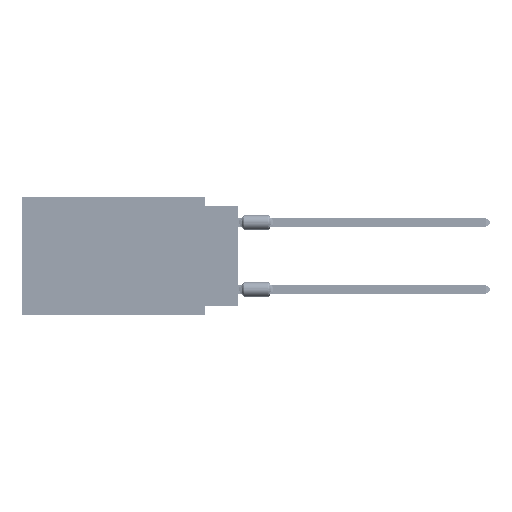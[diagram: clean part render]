
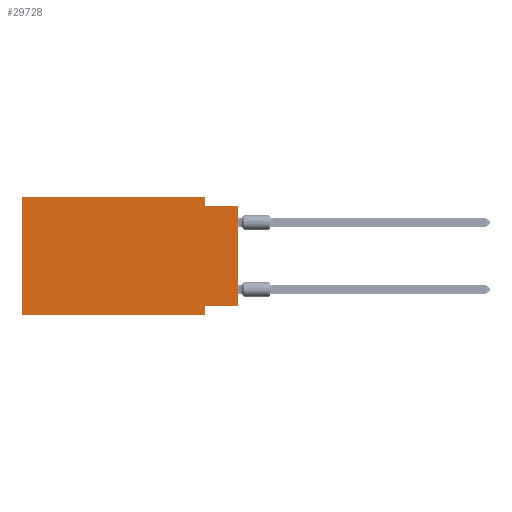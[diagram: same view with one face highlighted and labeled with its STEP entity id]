
A CAD part, left-side view. The second image highlights one B-rep face of the part: STEP entity #29728.
In plain terms, the highlighted planar face has unit normal (-1, 0, 0).
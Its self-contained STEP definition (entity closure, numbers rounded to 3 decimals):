
#1535 = VECTOR ( 'NONE', #17177, 1000. ) ;
#1628 = VECTOR ( 'NONE', #31292, 1000. ) ;
#6155 = DIRECTION ( 'NONE',  ( 0., 1., 0. ) ) ;
#7328 = LINE ( 'NONE', #43851, #18279 ) ;
#7484 = CARTESIAN_POINT ( 'NONE',  ( 0., 0., -0.635 ) ) ;
#7489 = LINE ( 'NONE', #72980, #1628 ) ;
#8551 = LINE ( 'NONE', #26423, #54644 ) ;
#9757 = VERTEX_POINT ( 'NONE', #61402 ) ;
#10589 = CARTESIAN_POINT ( 'NONE',  ( 0., 16.383, -8.89 ) ) ;
#12714 = ORIENTED_EDGE ( 'NONE', *, *, #69511, .F. ) ;
#13499 = VERTEX_POINT ( 'NONE', #23601 ) ;
#14620 = CARTESIAN_POINT ( 'NONE',  ( 0., 2.54, -8.255 ) ) ;
#14882 = PLANE ( 'NONE',  #59758 ) ;
#16758 = VERTEX_POINT ( 'NONE', #65951 ) ;
#16774 = VERTEX_POINT ( 'NONE', #60002 ) ;
#17177 = DIRECTION ( 'NONE',  ( 0., 0., 1. ) ) ;
#18279 = VECTOR ( 'NONE', #6155, 1000. ) ;
#19042 = EDGE_CURVE ( 'NONE', #13499, #16774, #39301, .T. ) ;
#19357 = ORIENTED_EDGE ( 'NONE', *, *, #62565, .F. ) ;
#20249 = DIRECTION ( 'NONE',  ( 0., 0., 1. ) ) ;
#22087 = VERTEX_POINT ( 'NONE', #34062 ) ;
#23601 = CARTESIAN_POINT ( 'NONE',  ( 0., 2.54, 0. ) ) ;
#24843 = EDGE_CURVE ( 'NONE', #33202, #16758, #37282, .T. ) ;
#26423 = CARTESIAN_POINT ( 'NONE',  ( 0., 2.54, -8.89 ) ) ;
#27209 = DIRECTION ( 'NONE',  ( 0., 0., -1. ) ) ;
#29728 = ADVANCED_FACE ( 'NONE', ( #76386 ), #14882, .F. ) ;
#31292 = DIRECTION ( 'NONE',  ( 0., -1., 0. ) ) ;
#33150 = DIRECTION ( 'NONE',  ( 1., 0., 0. ) ) ;
#33202 = VERTEX_POINT ( 'NONE', #10589 ) ;
#34062 = CARTESIAN_POINT ( 'NONE',  ( 0., 16.383, 0. ) ) ;
#34700 = ORIENTED_EDGE ( 'NONE', *, *, #24843, .T. ) ;
#37282 = LINE ( 'NONE', #49174, #55577 ) ;
#38123 = CARTESIAN_POINT ( 'NONE',  ( 0., 16.383, 0. ) ) ;
#38376 = VECTOR ( 'NONE', #38894, 1000. ) ;
#38894 = DIRECTION ( 'NONE',  ( 0., -1., 0. ) ) ;
#39301 = LINE ( 'NONE', #50836, #75336 ) ;
#39895 = CARTESIAN_POINT ( 'NONE',  ( 0., 16.383, 0. ) ) ;
#42739 = ORIENTED_EDGE ( 'NONE', *, *, #52417, .F. ) ;
#43851 = CARTESIAN_POINT ( 'NONE',  ( 0., 0., -8.255 ) ) ;
#43977 = EDGE_CURVE ( 'NONE', #16774, #49335, #7489, .T. ) ;
#46890 = ORIENTED_EDGE ( 'NONE', *, *, #19042, .F. ) ;
#47357 = LINE ( 'NONE', #71553, #1535 ) ;
#49139 = VECTOR ( 'NONE', #20249, 1000. ) ;
#49174 = CARTESIAN_POINT ( 'NONE',  ( 0., 16.383, -8.89 ) ) ;
#49312 = ORIENTED_EDGE ( 'NONE', *, *, #43977, .F. ) ;
#49335 = VERTEX_POINT ( 'NONE', #7484 ) ;
#50636 = DIRECTION ( 'NONE',  ( 0., 0., -1. ) ) ;
#50836 = CARTESIAN_POINT ( 'NONE',  ( 0., 2.54, 0. ) ) ;
#52417 = EDGE_CURVE ( 'NONE', #22087, #13499, #69056, .T. ) ;
#54644 = VECTOR ( 'NONE', #27209, 1000. ) ;
#55577 = VECTOR ( 'NONE', #62272, 1000. ) ;
#58422 = EDGE_CURVE ( 'NONE', #9757, #49335, #74616, .T. ) ;
#59758 = AXIS2_PLACEMENT_3D ( 'NONE', #39895, #33150, #50636 ) ;
#60002 = CARTESIAN_POINT ( 'NONE',  ( 0., 2.54, -0.635 ) ) ;
#61402 = CARTESIAN_POINT ( 'NONE',  ( 0., 0., -8.255 ) ) ;
#62272 = DIRECTION ( 'NONE',  ( 0., -1., 0. ) ) ;
#62565 = EDGE_CURVE ( 'NONE', #73597, #16758, #8551, .T. ) ;
#63499 = CARTESIAN_POINT ( 'NONE',  ( 0., 0., 0. ) ) ;
#65951 = CARTESIAN_POINT ( 'NONE',  ( 0., 2.54, -8.89 ) ) ;
#66998 = EDGE_CURVE ( 'NONE', #33202, #22087, #47357, .T. ) ;
#67064 = EDGE_LOOP ( 'NONE', ( #73533, #49312, #46890, #42739, #77985, #34700, #19357, #12714 ) ) ;
#69056 = LINE ( 'NONE', #38123, #38376 ) ;
#69511 = EDGE_CURVE ( 'NONE', #9757, #73597, #7328, .T. ) ;
#71553 = CARTESIAN_POINT ( 'NONE',  ( 0., 16.383, 0. ) ) ;
#72980 = CARTESIAN_POINT ( 'NONE',  ( 0., 0., -0.635 ) ) ;
#73533 = ORIENTED_EDGE ( 'NONE', *, *, #58422, .T. ) ;
#73597 = VERTEX_POINT ( 'NONE', #14620 ) ;
#74616 = LINE ( 'NONE', #63499, #49139 ) ;
#75030 = DIRECTION ( 'NONE',  ( 0., 0., -1. ) ) ;
#75336 = VECTOR ( 'NONE', #75030, 1000. ) ;
#76386 = FACE_OUTER_BOUND ( 'NONE', #67064, .T. ) ;
#77985 = ORIENTED_EDGE ( 'NONE', *, *, #66998, .F. ) ;
